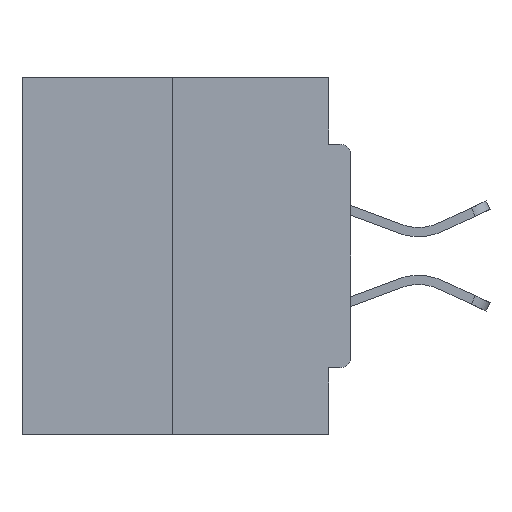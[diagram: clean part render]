
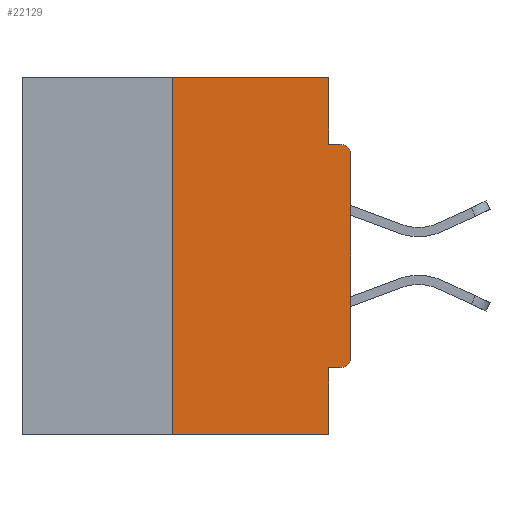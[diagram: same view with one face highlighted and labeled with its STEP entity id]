
A CAD part, left-side view. The second image highlights one B-rep face of the part: STEP entity #22129.
In plain terms, the highlighted planar face has unit normal (-1, 0, 0).
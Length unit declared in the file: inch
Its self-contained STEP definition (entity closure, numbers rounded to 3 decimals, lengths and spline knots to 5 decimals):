
#299 = DIRECTION ( 'NONE',  ( 1., 0., 0. ) ) ;
#344 = LINE ( 'NONE', #25565, #36597 ) ;
#1162 = DIRECTION ( 'NONE',  ( -1., 0., 0. ) ) ;
#1702 = VECTOR ( 'NONE', #10161, 39.37008 ) ;
#1796 = EDGE_CURVE ( 'NONE', #13942, #36383, #6272, .T. ) ;
#2756 = LINE ( 'NONE', #6206, #6845 ) ;
#2828 = CARTESIAN_POINT ( 'NONE',  ( 0., 0.015, -0.1085 ) ) ;
#2977 = EDGE_CURVE ( 'NONE', #25398, #27530, #11923, .T. ) ;
#3422 = DIRECTION ( 'NONE',  ( 0., 1., 0. ) ) ;
#3697 = EDGE_CURVE ( 'NONE', #36383, #25398, #35560, .T. ) ;
#3851 = AXIS2_PLACEMENT_3D ( 'NONE', #12748, #1162, #10002 ) ;
#4368 = EDGE_LOOP ( 'NONE', ( #18223, #20031, #7213, #33007, #30441, #9630, #9367, #16970, #34630, #14817 ) ) ;
#5064 = CIRCLE ( 'NONE', #3851, 0.015 ) ;
#5198 = DIRECTION ( 'NONE',  ( 0., -1., 0. ) ) ;
#6071 = VECTOR ( 'NONE', #32649, 39.37008 ) ;
#6206 = CARTESIAN_POINT ( 'NONE',  ( 0., 0., -0.4065 ) ) ;
#6272 = LINE ( 'NONE', #6690, #34462 ) ;
#6400 = CARTESIAN_POINT ( 'NONE',  ( 0., 0.25, -0.5 ) ) ;
#6412 = CARTESIAN_POINT ( 'NONE',  ( 0., 0.015, -0.4065 ) ) ;
#6690 = CARTESIAN_POINT ( 'NONE',  ( 0., 0.25, 0. ) ) ;
#6845 = VECTOR ( 'NONE', #3422, 39.37008 ) ;
#7157 = CARTESIAN_POINT ( 'NONE',  ( 0., 0.46, 0. ) ) ;
#7213 = ORIENTED_EDGE ( 'NONE', *, *, #8487, .T. ) ;
#7587 = FACE_OUTER_BOUND ( 'NONE', #4368, .T. ) ;
#8487 = EDGE_CURVE ( 'NONE', #13942, #13569, #16986, .T. ) ;
#8752 = EDGE_CURVE ( 'NONE', #27530, #33197, #344, .T. ) ;
#9153 = CARTESIAN_POINT ( 'NONE',  ( 0., 0.031, -0.4065 ) ) ;
#9367 = ORIENTED_EDGE ( 'NONE', *, *, #33737, .T. ) ;
#9630 = ORIENTED_EDGE ( 'NONE', *, *, #31743, .T. ) ;
#10002 = DIRECTION ( 'NONE',  ( 0., 0., -1. ) ) ;
#10161 = DIRECTION ( 'NONE',  ( 0., -1., 0. ) ) ;
#10769 = EDGE_CURVE ( 'NONE', #18163, #33197, #33762, .T. ) ;
#10889 = VERTEX_POINT ( 'NONE', #9153 ) ;
#10959 = CARTESIAN_POINT ( 'NONE',  ( 0., 0.015, -0.0935 ) ) ;
#11412 = DIRECTION ( 'NONE',  ( 0., 0., -1. ) ) ;
#11923 = LINE ( 'NONE', #18818, #6071 ) ;
#12148 = VERTEX_POINT ( 'NONE', #26387 ) ;
#12748 = CARTESIAN_POINT ( 'NONE',  ( 0., 0.015, -0.3915 ) ) ;
#13012 = CARTESIAN_POINT ( 'NONE',  ( 0., 0.25, 0. ) ) ;
#13569 = VERTEX_POINT ( 'NONE', #13679 ) ;
#13679 = CARTESIAN_POINT ( 'NONE',  ( 0., 0.031, -0.5 ) ) ;
#13942 = VERTEX_POINT ( 'NONE', #6400 ) ;
#14817 = ORIENTED_EDGE ( 'NONE', *, *, #2977, .F. ) ;
#15483 = VERTEX_POINT ( 'NONE', #6412 ) ;
#15853 = EDGE_CURVE ( 'NONE', #15483, #10889, #2756, .T. ) ;
#16970 = ORIENTED_EDGE ( 'NONE', *, *, #10769, .T. ) ;
#16986 = LINE ( 'NONE', #32710, #1702 ) ;
#17004 = DIRECTION ( 'NONE',  ( 0., 0., -1. ) ) ;
#17116 = CARTESIAN_POINT ( 'NONE',  ( 0., 0.46, 0. ) ) ;
#17216 = CARTESIAN_POINT ( 'NONE',  ( 0., 0.031, 0. ) ) ;
#17790 = VECTOR ( 'NONE', #19976, 39.37008 ) ;
#18163 = VERTEX_POINT ( 'NONE', #35449 ) ;
#18202 = DIRECTION ( 'NONE',  ( 0., 0., 1. ) ) ;
#18223 = ORIENTED_EDGE ( 'NONE', *, *, #3697, .F. ) ;
#18818 = CARTESIAN_POINT ( 'NONE',  ( 0., 0.031, 0. ) ) ;
#19300 = AXIS2_PLACEMENT_3D ( 'NONE', #17116, #299, #17004 ) ;
#19975 = DIRECTION ( 'NONE',  ( 0., -1., 0. ) ) ;
#19976 = DIRECTION ( 'NONE',  ( 0., 0., -1. ) ) ;
#20031 = ORIENTED_EDGE ( 'NONE', *, *, #1796, .F. ) ;
#20919 = LINE ( 'NONE', #25682, #17790 ) ;
#22129 = ADVANCED_FACE ( 'NONE', ( #7587 ), #31316, .F. ) ;
#23257 = CARTESIAN_POINT ( 'NONE',  ( 0., 0.031, -0.0935 ) ) ;
#24907 = LINE ( 'NONE', #32295, #33830 ) ;
#25398 = VERTEX_POINT ( 'NONE', #17216 ) ;
#25565 = CARTESIAN_POINT ( 'NONE',  ( 0., 0., -0.0935 ) ) ;
#25682 = CARTESIAN_POINT ( 'NONE',  ( 0., 0.031, -0.5 ) ) ;
#26387 = CARTESIAN_POINT ( 'NONE',  ( 0., 0., -0.3915 ) ) ;
#27062 = VECTOR ( 'NONE', #5198, 39.37008 ) ;
#27530 = VERTEX_POINT ( 'NONE', #23257 ) ;
#28301 = AXIS2_PLACEMENT_3D ( 'NONE', #2828, #28504, #11412 ) ;
#28504 = DIRECTION ( 'NONE',  ( -1., 0., 0. ) ) ;
#30441 = ORIENTED_EDGE ( 'NONE', *, *, #15853, .F. ) ;
#31316 = PLANE ( 'NONE',  #19300 ) ;
#31743 = EDGE_CURVE ( 'NONE', #15483, #12148, #5064, .T. ) ;
#32295 = CARTESIAN_POINT ( 'NONE',  ( 0., 0., 0. ) ) ;
#32649 = DIRECTION ( 'NONE',  ( 0., 0., -1. ) ) ;
#32710 = CARTESIAN_POINT ( 'NONE',  ( 0., 0.46, -0.5 ) ) ;
#33007 = ORIENTED_EDGE ( 'NONE', *, *, #33634, .F. ) ;
#33197 = VERTEX_POINT ( 'NONE', #10959 ) ;
#33634 = EDGE_CURVE ( 'NONE', #10889, #13569, #20919, .T. ) ;
#33737 = EDGE_CURVE ( 'NONE', #12148, #18163, #24907, .T. ) ;
#33762 = CIRCLE ( 'NONE', #28301, 0.015 ) ;
#33830 = VECTOR ( 'NONE', #34690, 39.37008 ) ;
#34462 = VECTOR ( 'NONE', #18202, 39.37008 ) ;
#34630 = ORIENTED_EDGE ( 'NONE', *, *, #8752, .F. ) ;
#34690 = DIRECTION ( 'NONE',  ( 0., 0., 1. ) ) ;
#35449 = CARTESIAN_POINT ( 'NONE',  ( 0., 0., -0.1085 ) ) ;
#35560 = LINE ( 'NONE', #7157, #27062 ) ;
#36383 = VERTEX_POINT ( 'NONE', #13012 ) ;
#36597 = VECTOR ( 'NONE', #19975, 39.37008 ) ;
